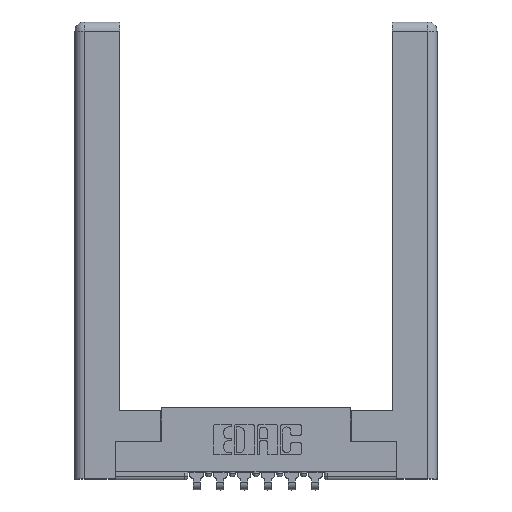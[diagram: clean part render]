
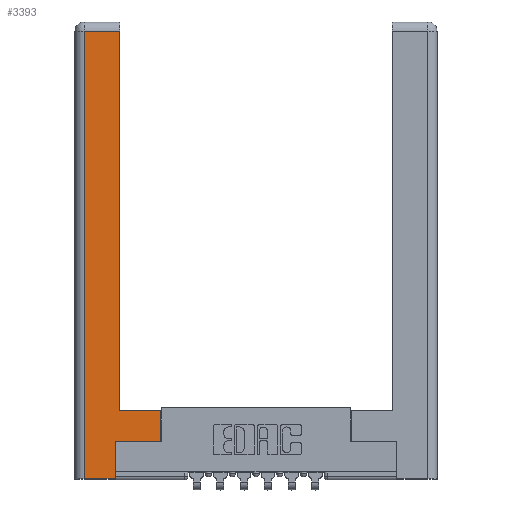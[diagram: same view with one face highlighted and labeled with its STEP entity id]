
A CAD part, top view. The second image highlights one B-rep face of the part: STEP entity #3393.
In plain terms, the highlighted planar face has unit normal (0, 0, 1).
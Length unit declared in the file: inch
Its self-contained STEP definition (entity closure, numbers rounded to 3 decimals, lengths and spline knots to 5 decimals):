
#2 = CARTESIAN_POINT ( 'NONE',  ( 0.0615, 2.94, 0. ) ) ;
#305 = PLANE ( 'NONE',  #2264 ) ;
#326 = LINE ( 'NONE', #9941, #10466 ) ;
#353 = VERTEX_POINT ( 'NONE', #1021 ) ;
#387 = VERTEX_POINT ( 'NONE', #11510 ) ;
#416 = CARTESIAN_POINT ( 'NONE',  ( 0.295, 0.45, 0. ) ) ;
#945 = CARTESIAN_POINT ( 'NONE',  ( 0.295, 3., 0. ) ) ;
#1021 = CARTESIAN_POINT ( 'NONE',  ( 0.295, 0.45, 0. ) ) ;
#1266 = VERTEX_POINT ( 'NONE', #10213 ) ;
#1302 = CARTESIAN_POINT ( 'NONE',  ( 0.565, 0.245, 0. ) ) ;
#1572 = DIRECTION ( 'NONE',  ( 0., -1., 0. ) ) ;
#1722 = LINE ( 'NONE', #10281, #3857 ) ;
#1870 = VECTOR ( 'NONE', #3858, 39.37008 ) ;
#2264 = AXIS2_PLACEMENT_3D ( 'NONE', #10675, #6092, #4977 ) ;
#2385 = DIRECTION ( 'NONE',  ( 0., 1., 0. ) ) ;
#2519 = EDGE_CURVE ( 'NONE', #387, #9239, #9018, .T. ) ;
#2712 = ORIENTED_EDGE ( 'NONE', *, *, #4967, .T. ) ;
#3153 = EDGE_CURVE ( 'NONE', #5197, #10667, #9566, .T. ) ;
#3393 = ADVANCED_FACE ( 'NONE', ( #6848 ), #305, .F. ) ;
#3398 = CARTESIAN_POINT ( 'NONE',  ( 0.295, 2.94, 0. ) ) ;
#3483 = CARTESIAN_POINT ( 'NONE',  ( 0.0615, 0., 0. ) ) ;
#3748 = VERTEX_POINT ( 'NONE', #11808 ) ;
#3857 = VECTOR ( 'NONE', #11194, 39.37008 ) ;
#3858 = DIRECTION ( 'NONE',  ( -1., 0., 0. ) ) ;
#3954 = EDGE_CURVE ( 'NONE', #3748, #5333, #1722, .T. ) ;
#4037 = ORIENTED_EDGE ( 'NONE', *, *, #6668, .T. ) ;
#4177 = EDGE_CURVE ( 'NONE', #9239, #1266, #326, .T. ) ;
#4198 = VECTOR ( 'NONE', #1572, 39.37008 ) ;
#4217 = CARTESIAN_POINT ( 'NONE',  ( 0.0615, 2.94, 0. ) ) ;
#4726 = DIRECTION ( 'NONE',  ( 0., 1., 0. ) ) ;
#4769 = CARTESIAN_POINT ( 'NONE',  ( 0.265, 0., 0. ) ) ;
#4967 = EDGE_CURVE ( 'NONE', #353, #5197, #5667, .T. ) ;
#4977 = DIRECTION ( 'NONE',  ( -1., 0., 0. ) ) ;
#5107 = LINE ( 'NONE', #3483, #4198 ) ;
#5197 = VERTEX_POINT ( 'NONE', #3398 ) ;
#5333 = VERTEX_POINT ( 'NONE', #4769 ) ;
#5667 = LINE ( 'NONE', #945, #9682 ) ;
#5710 = VECTOR ( 'NONE', #8143, 39.37008 ) ;
#6052 = EDGE_CURVE ( 'NONE', #1266, #353, #11713, .T. ) ;
#6092 = DIRECTION ( 'NONE',  ( 0., 0., -1. ) ) ;
#6132 = CARTESIAN_POINT ( 'NONE',  ( 0.265, 0.245, 0. ) ) ;
#6271 = ORIENTED_EDGE ( 'NONE', *, *, #6052, .T. ) ;
#6304 = ORIENTED_EDGE ( 'NONE', *, *, #2519, .T. ) ;
#6309 = DIRECTION ( 'NONE',  ( 1., 0., 0. ) ) ;
#6625 = VECTOR ( 'NONE', #6309, 39.37008 ) ;
#6668 = EDGE_CURVE ( 'NONE', #5333, #387, #8278, .T. ) ;
#6848 = FACE_OUTER_BOUND ( 'NONE', #7762, .T. ) ;
#7762 = EDGE_LOOP ( 'NONE', ( #2712, #10260, #10909, #9026, #4037, #6304, #10053, #6271 ) ) ;
#8143 = DIRECTION ( 'NONE',  ( 0., 1., 0. ) ) ;
#8278 = LINE ( 'NONE', #6132, #5710 ) ;
#8747 = DIRECTION ( 'NONE',  ( -1., 0., 0. ) ) ;
#9018 = LINE ( 'NONE', #9339, #6625 ) ;
#9026 = ORIENTED_EDGE ( 'NONE', *, *, #3954, .T. ) ;
#9239 = VERTEX_POINT ( 'NONE', #1302 ) ;
#9339 = CARTESIAN_POINT ( 'NONE',  ( 0.565, 0.245, 0. ) ) ;
#9566 = LINE ( 'NONE', #2, #1870 ) ;
#9682 = VECTOR ( 'NONE', #4726, 39.37008 ) ;
#9711 = VECTOR ( 'NONE', #8747, 39.37008 ) ;
#9941 = CARTESIAN_POINT ( 'NONE',  ( 0.565, 0.45, 0. ) ) ;
#10053 = ORIENTED_EDGE ( 'NONE', *, *, #4177, .T. ) ;
#10213 = CARTESIAN_POINT ( 'NONE',  ( 0.565, 0.45, 0. ) ) ;
#10260 = ORIENTED_EDGE ( 'NONE', *, *, #3153, .T. ) ;
#10281 = CARTESIAN_POINT ( 'NONE',  ( 0.265, 0., 0. ) ) ;
#10466 = VECTOR ( 'NONE', #2385, 39.37008 ) ;
#10667 = VERTEX_POINT ( 'NONE', #4217 ) ;
#10675 = CARTESIAN_POINT ( 'NONE',  ( 0., 0., 0. ) ) ;
#10909 = ORIENTED_EDGE ( 'NONE', *, *, #11479, .T. ) ;
#11194 = DIRECTION ( 'NONE',  ( 1., 0., 0. ) ) ;
#11479 = EDGE_CURVE ( 'NONE', #10667, #3748, #5107, .T. ) ;
#11510 = CARTESIAN_POINT ( 'NONE',  ( 0.265, 0.245, 0. ) ) ;
#11713 = LINE ( 'NONE', #416, #9711 ) ;
#11808 = CARTESIAN_POINT ( 'NONE',  ( 0.0615, 0., 0. ) ) ;
